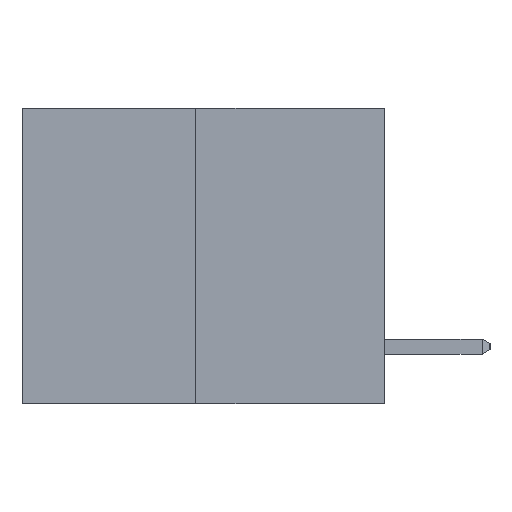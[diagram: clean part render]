
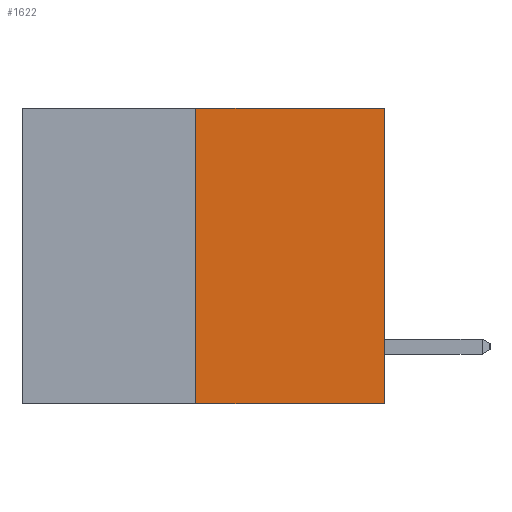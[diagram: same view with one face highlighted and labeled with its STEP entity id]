
A CAD part, left-side view. The second image highlights one B-rep face of the part: STEP entity #1622.
In plain terms, the highlighted planar face has unit normal (-1, 0, 0).
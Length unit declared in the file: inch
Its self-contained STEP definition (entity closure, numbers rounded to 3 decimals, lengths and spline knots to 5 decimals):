
#70 = DIRECTION ( 'NONE',  ( 1., 0., 0. ) ) ;
#75 = VERTEX_POINT ( 'NONE', #12755 ) ;
#1622 = ADVANCED_FACE ( 'NONE', ( #13935 ), #17256, .F. ) ;
#1775 = ORIENTED_EDGE ( 'NONE', *, *, #18179, .F. ) ;
#1780 = CARTESIAN_POINT ( 'NONE',  ( 0., 0.6, 0. ) ) ;
#2329 = EDGE_CURVE ( 'NONE', #24919, #12878, #19348, .T. ) ;
#3156 = LINE ( 'NONE', #19829, #10378 ) ;
#3885 = AXIS2_PLACEMENT_3D ( 'NONE', #1780, #70, #13545 ) ;
#4288 = EDGE_CURVE ( 'NONE', #12878, #75, #11054, .T. ) ;
#5534 = VERTEX_POINT ( 'NONE', #22590 ) ;
#7488 = EDGE_CURVE ( 'NONE', #5534, #75, #14407, .T. ) ;
#7967 = ORIENTED_EDGE ( 'NONE', *, *, #7488, .F. ) ;
#9543 = CARTESIAN_POINT ( 'NONE',  ( 0., 0., 0. ) ) ;
#10101 = DIRECTION ( 'NONE',  ( 0., -1., 0. ) ) ;
#10378 = VECTOR ( 'NONE', #19914, 39.37008 ) ;
#11054 = LINE ( 'NONE', #9543, #23428 ) ;
#11059 = ORIENTED_EDGE ( 'NONE', *, *, #2329, .T. ) ;
#11270 = CARTESIAN_POINT ( 'NONE',  ( 0., 0., -0.49 ) ) ;
#12413 = VECTOR ( 'NONE', #22256, 39.37008 ) ;
#12755 = CARTESIAN_POINT ( 'NONE',  ( 0., 0., 0. ) ) ;
#12878 = VERTEX_POINT ( 'NONE', #11270 ) ;
#13258 = DIRECTION ( 'NONE',  ( 0., 0., 1. ) ) ;
#13545 = DIRECTION ( 'NONE',  ( 0., 0., -1. ) ) ;
#13935 = FACE_OUTER_BOUND ( 'NONE', #20358, .T. ) ;
#14198 = CARTESIAN_POINT ( 'NONE',  ( 0., 0.312, -0.49 ) ) ;
#14407 = LINE ( 'NONE', #19628, #22233 ) ;
#17256 = PLANE ( 'NONE',  #3885 ) ;
#17267 = ORIENTED_EDGE ( 'NONE', *, *, #4288, .T. ) ;
#18179 = EDGE_CURVE ( 'NONE', #24919, #5534, #3156, .T. ) ;
#19348 = LINE ( 'NONE', #24444, #12413 ) ;
#19628 = CARTESIAN_POINT ( 'NONE',  ( 0., 0.6, 0. ) ) ;
#19829 = CARTESIAN_POINT ( 'NONE',  ( 0., 0.312, -0.49 ) ) ;
#19914 = DIRECTION ( 'NONE',  ( 0., 0., 1. ) ) ;
#20358 = EDGE_LOOP ( 'NONE', ( #1775, #11059, #17267, #7967 ) ) ;
#22233 = VECTOR ( 'NONE', #10101, 39.37008 ) ;
#22256 = DIRECTION ( 'NONE',  ( 0., -1., 0. ) ) ;
#22590 = CARTESIAN_POINT ( 'NONE',  ( 0., 0.312, 0. ) ) ;
#23428 = VECTOR ( 'NONE', #13258, 39.37008 ) ;
#24444 = CARTESIAN_POINT ( 'NONE',  ( 0., 0.6, -0.49 ) ) ;
#24919 = VERTEX_POINT ( 'NONE', #14198 ) ;
